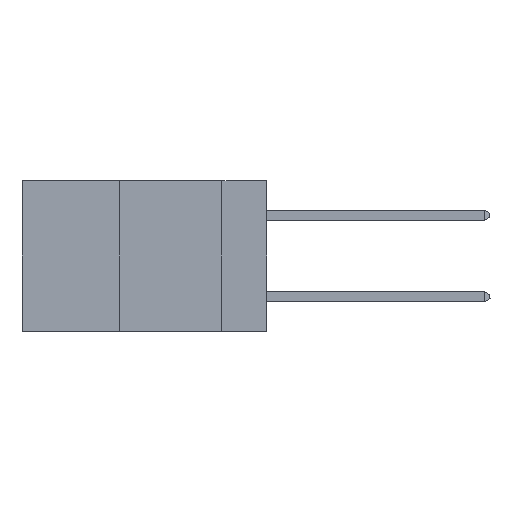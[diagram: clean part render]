
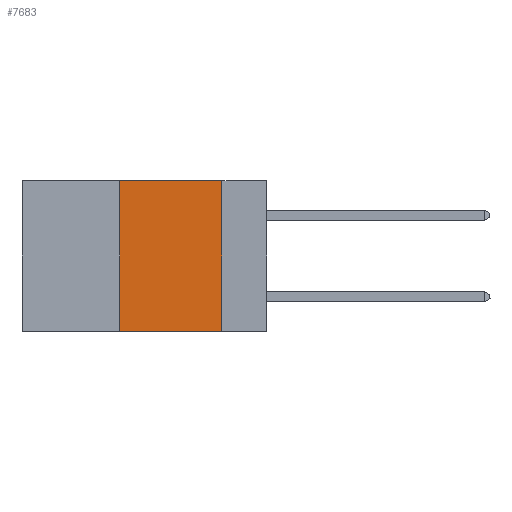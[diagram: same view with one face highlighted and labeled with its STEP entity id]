
A CAD part, left-side view. The second image highlights one B-rep face of the part: STEP entity #7683.
In plain terms, the highlighted planar face has unit normal (-1, 0, 0).
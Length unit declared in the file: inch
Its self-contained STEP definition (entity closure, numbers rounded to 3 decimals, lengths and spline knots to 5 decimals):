
#779 = VERTEX_POINT ( 'NONE', #10916 ) ;
#1650 = CARTESIAN_POINT ( 'NONE',  ( 0., 0.6, 0. ) ) ;
#2188 = PLANE ( 'NONE',  #9542 ) ;
#2388 = CARTESIAN_POINT ( 'NONE',  ( 0., 0.6, 0. ) ) ;
#3118 = VERTEX_POINT ( 'NONE', #26725 ) ;
#3135 = VERTEX_POINT ( 'NONE', #3512 ) ;
#3392 = DIRECTION ( 'NONE',  ( 0., 0., -1. ) ) ;
#3512 = CARTESIAN_POINT ( 'NONE',  ( 0., 0.11, 0. ) ) ;
#6262 = DIRECTION ( 'NONE',  ( 0., -1., 0. ) ) ;
#7683 = ADVANCED_FACE ( 'NONE', ( #11072 ), #2188, .F. ) ;
#8395 = CARTESIAN_POINT ( 'NONE',  ( 0., 0.36, 0. ) ) ;
#8745 = EDGE_CURVE ( 'NONE', #779, #11538, #20011, .T. ) ;
#9542 = AXIS2_PLACEMENT_3D ( 'NONE', #2388, #16053, #13633 ) ;
#9722 = ORIENTED_EDGE ( 'NONE', *, *, #15724, .F. ) ;
#10916 = CARTESIAN_POINT ( 'NONE',  ( 0., 0.36, -0.37 ) ) ;
#11072 = FACE_OUTER_BOUND ( 'NONE', #22005, .T. ) ;
#11417 = DIRECTION ( 'NONE',  ( 0., 0., 1. ) ) ;
#11538 = VERTEX_POINT ( 'NONE', #8395 ) ;
#11908 = CARTESIAN_POINT ( 'NONE',  ( 0., 0.11, 0. ) ) ;
#13633 = DIRECTION ( 'NONE',  ( 0., 0., -1. ) ) ;
#13741 = LINE ( 'NONE', #11908, #25234 ) ;
#15724 = EDGE_CURVE ( 'NONE', #11538, #3135, #26015, .T. ) ;
#16053 = DIRECTION ( 'NONE',  ( 1., 0., 0. ) ) ;
#17438 = EDGE_CURVE ( 'NONE', #779, #3118, #18022, .T. ) ;
#18022 = LINE ( 'NONE', #26406, #25172 ) ;
#18994 = ORIENTED_EDGE ( 'NONE', *, *, #17438, .T. ) ;
#19475 = DIRECTION ( 'NONE',  ( 0., -1., 0. ) ) ;
#20011 = LINE ( 'NONE', #20689, #28278 ) ;
#20133 = ORIENTED_EDGE ( 'NONE', *, *, #8745, .F. ) ;
#20689 = CARTESIAN_POINT ( 'NONE',  ( 0., 0.36, 0. ) ) ;
#20995 = EDGE_CURVE ( 'NONE', #3135, #3118, #13741, .T. ) ;
#22005 = EDGE_LOOP ( 'NONE', ( #26777, #9722, #20133, #18994 ) ) ;
#25172 = VECTOR ( 'NONE', #19475, 39.37008 ) ;
#25234 = VECTOR ( 'NONE', #3392, 39.37008 ) ;
#26015 = LINE ( 'NONE', #1650, #27141 ) ;
#26406 = CARTESIAN_POINT ( 'NONE',  ( 0., 0.6, -0.37 ) ) ;
#26725 = CARTESIAN_POINT ( 'NONE',  ( 0., 0.11, -0.37 ) ) ;
#26777 = ORIENTED_EDGE ( 'NONE', *, *, #20995, .F. ) ;
#27141 = VECTOR ( 'NONE', #6262, 39.37008 ) ;
#28278 = VECTOR ( 'NONE', #11417, 39.37008 ) ;
